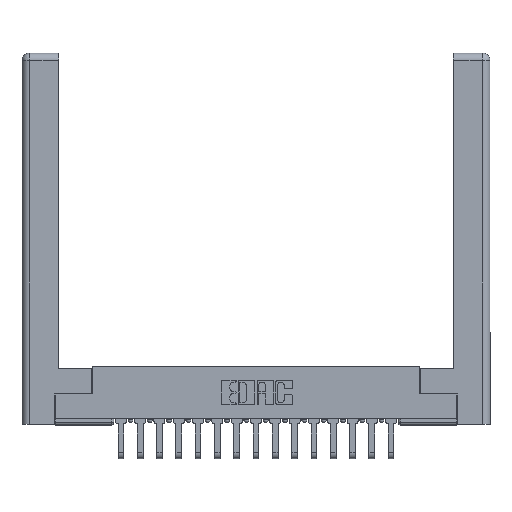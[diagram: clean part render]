
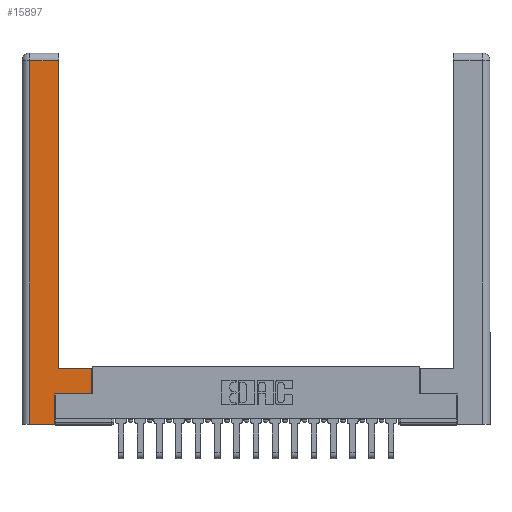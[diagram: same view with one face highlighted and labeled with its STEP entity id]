
A CAD part, top view. The second image highlights one B-rep face of the part: STEP entity #15897.
In plain terms, the highlighted planar face has unit normal (0, 0, 1).
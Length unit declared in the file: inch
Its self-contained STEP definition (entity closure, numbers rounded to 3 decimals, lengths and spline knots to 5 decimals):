
#290 = DIRECTION ( 'NONE',  ( 0., 1., 0. ) ) ;
#318 = VECTOR ( 'NONE', #10777, 39.37008 ) ;
#520 = CARTESIAN_POINT ( 'NONE',  ( 0.295, 0.45, 0. ) ) ;
#665 = VERTEX_POINT ( 'NONE', #14222 ) ;
#701 = FACE_OUTER_BOUND ( 'NONE', #8654, .T. ) ;
#815 = LINE ( 'NONE', #17271, #318 ) ;
#2283 = DIRECTION ( 'NONE',  ( 0., -1., 0. ) ) ;
#3291 = ORIENTED_EDGE ( 'NONE', *, *, #8215, .T. ) ;
#3739 = EDGE_CURVE ( 'NONE', #5138, #5018, #12200, .T. ) ;
#4278 = DIRECTION ( 'NONE',  ( -1., 0., 0. ) ) ;
#4325 = CARTESIAN_POINT ( 'NONE',  ( 0.265, 0., 0. ) ) ;
#4377 = LINE ( 'NONE', #16450, #20439 ) ;
#5018 = VERTEX_POINT ( 'NONE', #14931 ) ;
#5094 = EDGE_CURVE ( 'NONE', #12408, #5138, #4377, .T. ) ;
#5138 = VERTEX_POINT ( 'NONE', #520 ) ;
#5310 = CARTESIAN_POINT ( 'NONE',  ( 0.565, 0.245, 0. ) ) ;
#5339 = LINE ( 'NONE', #17612, #13332 ) ;
#5586 = ORIENTED_EDGE ( 'NONE', *, *, #15848, .T. ) ;
#5845 = VERTEX_POINT ( 'NONE', #6105 ) ;
#6105 = CARTESIAN_POINT ( 'NONE',  ( 0.0615, 2.94, 0. ) ) ;
#6611 = LINE ( 'NONE', #10047, #16310 ) ;
#6777 = AXIS2_PLACEMENT_3D ( 'NONE', #8195, #19730, #4278 ) ;
#6943 = VECTOR ( 'NONE', #290, 39.37008 ) ;
#7030 = VECTOR ( 'NONE', #9146, 39.37008 ) ;
#7766 = VECTOR ( 'NONE', #16468, 39.37008 ) ;
#8195 = CARTESIAN_POINT ( 'NONE',  ( 0., 0., 0. ) ) ;
#8215 = EDGE_CURVE ( 'NONE', #9913, #15203, #815, .T. ) ;
#8298 = EDGE_CURVE ( 'NONE', #665, #9913, #5339, .T. ) ;
#8555 = EDGE_CURVE ( 'NONE', #9525, #12408, #6611, .T. ) ;
#8654 = EDGE_LOOP ( 'NONE', ( #15061, #16642, #18670, #9358, #3291, #5586, #11223, #9841 ) ) ;
#9146 = DIRECTION ( 'NONE',  ( -1., 0., 0. ) ) ;
#9358 = ORIENTED_EDGE ( 'NONE', *, *, #8298, .T. ) ;
#9525 = VERTEX_POINT ( 'NONE', #17226 ) ;
#9841 = ORIENTED_EDGE ( 'NONE', *, *, #5094, .T. ) ;
#9913 = VERTEX_POINT ( 'NONE', #4325 ) ;
#10047 = CARTESIAN_POINT ( 'NONE',  ( 0.565, 0.45, 0. ) ) ;
#10290 = EDGE_CURVE ( 'NONE', #5018, #5845, #16245, .T. ) ;
#10777 = DIRECTION ( 'NONE',  ( 0., 1., 0. ) ) ;
#11223 = ORIENTED_EDGE ( 'NONE', *, *, #8555, .T. ) ;
#12200 = LINE ( 'NONE', #14583, #6943 ) ;
#12408 = VERTEX_POINT ( 'NONE', #17416 ) ;
#12671 = LINE ( 'NONE', #14934, #16155 ) ;
#12880 = DIRECTION ( 'NONE',  ( 0., 1., 0. ) ) ;
#13332 = VECTOR ( 'NONE', #14224, 39.37008 ) ;
#14000 = LINE ( 'NONE', #5310, #7766 ) ;
#14222 = CARTESIAN_POINT ( 'NONE',  ( 0.0615, 0., 0. ) ) ;
#14224 = DIRECTION ( 'NONE',  ( 1., 0., 0. ) ) ;
#14583 = CARTESIAN_POINT ( 'NONE',  ( 0.295, 3., 0. ) ) ;
#14850 = PLANE ( 'NONE',  #6777 ) ;
#14931 = CARTESIAN_POINT ( 'NONE',  ( 0.295, 2.94, 0. ) ) ;
#14934 = CARTESIAN_POINT ( 'NONE',  ( 0.0615, 0., 0. ) ) ;
#15061 = ORIENTED_EDGE ( 'NONE', *, *, #3739, .T. ) ;
#15203 = VERTEX_POINT ( 'NONE', #19398 ) ;
#15848 = EDGE_CURVE ( 'NONE', #15203, #9525, #14000, .T. ) ;
#15897 = ADVANCED_FACE ( 'NONE', ( #701 ), #14850, .F. ) ;
#16155 = VECTOR ( 'NONE', #2283, 39.37008 ) ;
#16245 = LINE ( 'NONE', #20404, #7030 ) ;
#16310 = VECTOR ( 'NONE', #12880, 39.37008 ) ;
#16382 = DIRECTION ( 'NONE',  ( -1., 0., 0. ) ) ;
#16450 = CARTESIAN_POINT ( 'NONE',  ( 0.295, 0.45, 0. ) ) ;
#16468 = DIRECTION ( 'NONE',  ( 1., 0., 0. ) ) ;
#16642 = ORIENTED_EDGE ( 'NONE', *, *, #10290, .T. ) ;
#17226 = CARTESIAN_POINT ( 'NONE',  ( 0.565, 0.245, 0. ) ) ;
#17271 = CARTESIAN_POINT ( 'NONE',  ( 0.265, 0.245, 0. ) ) ;
#17416 = CARTESIAN_POINT ( 'NONE',  ( 0.565, 0.45, 0. ) ) ;
#17612 = CARTESIAN_POINT ( 'NONE',  ( 0.265, 0., 0. ) ) ;
#18670 = ORIENTED_EDGE ( 'NONE', *, *, #20414, .T. ) ;
#19398 = CARTESIAN_POINT ( 'NONE',  ( 0.265, 0.245, 0. ) ) ;
#19730 = DIRECTION ( 'NONE',  ( 0., 0., -1. ) ) ;
#20404 = CARTESIAN_POINT ( 'NONE',  ( 0.0615, 2.94, 0. ) ) ;
#20414 = EDGE_CURVE ( 'NONE', #5845, #665, #12671, .T. ) ;
#20439 = VECTOR ( 'NONE', #16382, 39.37008 ) ;
